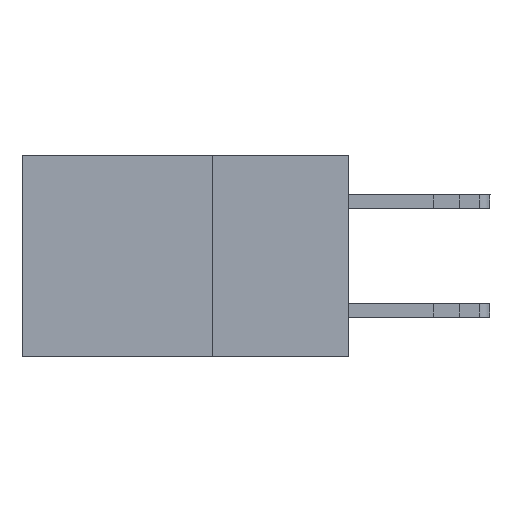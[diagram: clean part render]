
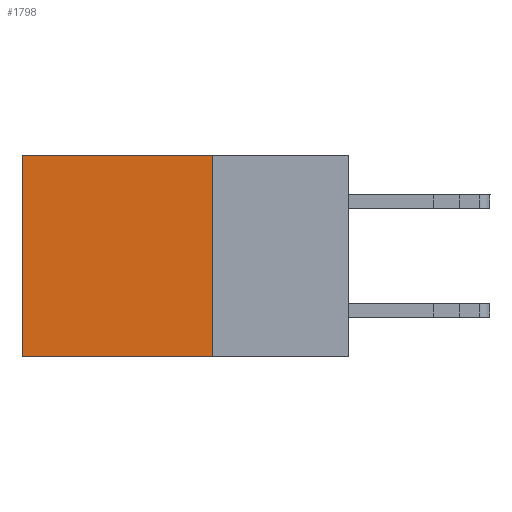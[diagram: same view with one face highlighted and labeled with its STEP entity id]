
A CAD part, left-side view. The second image highlights one B-rep face of the part: STEP entity #1798.
In plain terms, the highlighted planar face has unit normal (-1, 0, 0).
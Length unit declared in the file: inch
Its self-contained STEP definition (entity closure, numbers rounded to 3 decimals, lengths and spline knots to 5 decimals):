
#53 = VECTOR ( 'NONE', #8619, 39.37008 ) ;
#341 = VERTEX_POINT ( 'NONE', #1818 ) ;
#681 = CARTESIAN_POINT ( 'NONE',  ( 0.298, 0.6, 0. ) ) ;
#744 = PLANE ( 'NONE',  #11576 ) ;
#834 = FACE_OUTER_BOUND ( 'NONE', #3956, .T. ) ;
#1613 = CARTESIAN_POINT ( 'NONE',  ( 0.298, 0.25, 0. ) ) ;
#1798 = ADVANCED_FACE ( 'NONE', ( #834 ), #744, .F. ) ;
#1818 = CARTESIAN_POINT ( 'NONE',  ( 0.298, 0.25, -0.37 ) ) ;
#2098 = LINE ( 'NONE', #11440, #13421 ) ;
#2262 = DIRECTION ( 'NONE',  ( 1., 0., 0. ) ) ;
#2538 = LINE ( 'NONE', #10622, #8920 ) ;
#2585 = CARTESIAN_POINT ( 'NONE',  ( 0.298, 0.25, 0. ) ) ;
#3350 = DIRECTION ( 'NONE',  ( 0., 0., -1. ) ) ;
#3523 = DIRECTION ( 'NONE',  ( 0., 1., 0. ) ) ;
#3956 = EDGE_LOOP ( 'NONE', ( #16348, #6215, #7661, #10504 ) ) ;
#4501 = EDGE_CURVE ( 'NONE', #341, #16840, #2538, .T. ) ;
#6215 = ORIENTED_EDGE ( 'NONE', *, *, #4501, .F. ) ;
#7661 = ORIENTED_EDGE ( 'NONE', *, *, #14762, .F. ) ;
#8100 = VERTEX_POINT ( 'NONE', #2585 ) ;
#8619 = DIRECTION ( 'NONE',  ( 0., 0., -1. ) ) ;
#8920 = VECTOR ( 'NONE', #10709, 39.37008 ) ;
#9015 = CARTESIAN_POINT ( 'NONE',  ( 0.298, 0.25, 0. ) ) ;
#9971 = EDGE_CURVE ( 'NONE', #8100, #16904, #11542, .T. ) ;
#10504 = ORIENTED_EDGE ( 'NONE', *, *, #9971, .T. ) ;
#10525 = DIRECTION ( 'NONE',  ( 0., 0., -1. ) ) ;
#10622 = CARTESIAN_POINT ( 'NONE',  ( 0.298, 0.25, -0.37 ) ) ;
#10709 = DIRECTION ( 'NONE',  ( 0., 1., 0. ) ) ;
#11440 = CARTESIAN_POINT ( 'NONE',  ( 0.298, 0.6, 0. ) ) ;
#11542 = LINE ( 'NONE', #15684, #12116 ) ;
#11576 = AXIS2_PLACEMENT_3D ( 'NONE', #9015, #2262, #10525 ) ;
#12116 = VECTOR ( 'NONE', #3523, 39.37008 ) ;
#13421 = VECTOR ( 'NONE', #3350, 39.37008 ) ;
#13782 = LINE ( 'NONE', #1613, #53 ) ;
#14762 = EDGE_CURVE ( 'NONE', #8100, #341, #13782, .T. ) ;
#15430 = CARTESIAN_POINT ( 'NONE',  ( 0.298, 0.6, -0.37 ) ) ;
#15684 = CARTESIAN_POINT ( 'NONE',  ( 0.298, 0.25, 0. ) ) ;
#16348 = ORIENTED_EDGE ( 'NONE', *, *, #17297, .T. ) ;
#16840 = VERTEX_POINT ( 'NONE', #15430 ) ;
#16904 = VERTEX_POINT ( 'NONE', #681 ) ;
#17297 = EDGE_CURVE ( 'NONE', #16904, #16840, #2098, .T. ) ;
